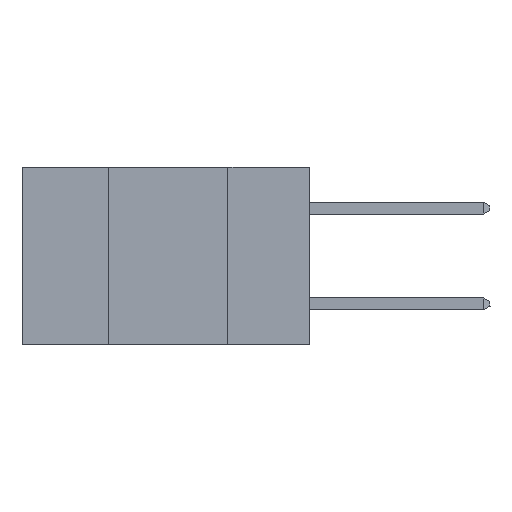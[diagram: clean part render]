
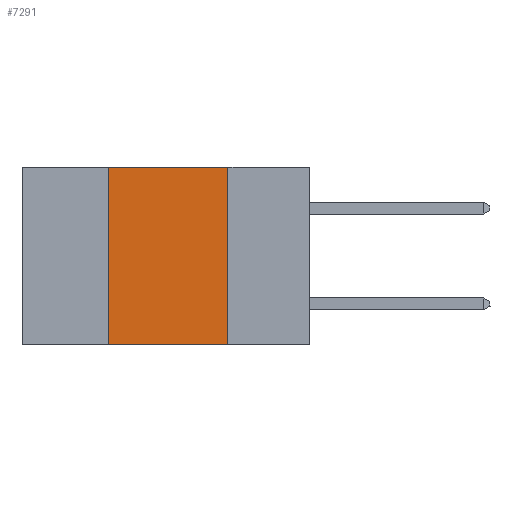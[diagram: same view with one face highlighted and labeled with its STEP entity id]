
A CAD part, left-side view. The second image highlights one B-rep face of the part: STEP entity #7291.
In plain terms, the highlighted planar face has unit normal (-1, 0, 0).
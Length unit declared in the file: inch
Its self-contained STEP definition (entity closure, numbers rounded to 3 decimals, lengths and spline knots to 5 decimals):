
#72 = AXIS2_PLACEMENT_3D ( 'NONE', #28577, #18499, #19022 ) ;
#2441 = VERTEX_POINT ( 'NONE', #14152 ) ;
#2989 = ORIENTED_EDGE ( 'NONE', *, *, #26535, .T. ) ;
#5085 = LINE ( 'NONE', #9541, #8541 ) ;
#5310 = DIRECTION ( 'NONE',  ( 0., -1., 0. ) ) ;
#5740 = VERTEX_POINT ( 'NONE', #23382 ) ;
#6994 = EDGE_CURVE ( 'NONE', #11502, #2441, #5085, .T. ) ;
#7291 = ADVANCED_FACE ( 'NONE', ( #26957 ), #26006, .F. ) ;
#7890 = LINE ( 'NONE', #20004, #15996 ) ;
#7970 = VECTOR ( 'NONE', #14049, 39.37008 ) ;
#8541 = VECTOR ( 'NONE', #21970, 39.37008 ) ;
#9541 = CARTESIAN_POINT ( 'NONE',  ( 0., 0.17, 0. ) ) ;
#9590 = VECTOR ( 'NONE', #28060, 39.37008 ) ;
#10100 = CARTESIAN_POINT ( 'NONE',  ( 0., 0.42, 0. ) ) ;
#11502 = VERTEX_POINT ( 'NONE', #21908 ) ;
#11761 = ORIENTED_EDGE ( 'NONE', *, *, #6994, .F. ) ;
#12871 = EDGE_LOOP ( 'NONE', ( #11761, #29913, #15161, #2989 ) ) ;
#13013 = LINE ( 'NONE', #10100, #9590 ) ;
#14049 = DIRECTION ( 'NONE',  ( 0., -1., 0. ) ) ;
#14152 = CARTESIAN_POINT ( 'NONE',  ( 0., 0.17, -0.37 ) ) ;
#15161 = ORIENTED_EDGE ( 'NONE', *, *, #21247, .F. ) ;
#15996 = VECTOR ( 'NONE', #5310, 39.37008 ) ;
#16060 = EDGE_CURVE ( 'NONE', #5740, #11502, #7890, .T. ) ;
#17569 = VERTEX_POINT ( 'NONE', #21531 ) ;
#18499 = DIRECTION ( 'NONE',  ( 1., 0., 0. ) ) ;
#19022 = DIRECTION ( 'NONE',  ( 0., 0., -1. ) ) ;
#20004 = CARTESIAN_POINT ( 'NONE',  ( 0., 0.6, 0. ) ) ;
#21247 = EDGE_CURVE ( 'NONE', #17569, #5740, #13013, .T. ) ;
#21531 = CARTESIAN_POINT ( 'NONE',  ( 0., 0.42, -0.37 ) ) ;
#21908 = CARTESIAN_POINT ( 'NONE',  ( 0., 0.17, 0. ) ) ;
#21970 = DIRECTION ( 'NONE',  ( 0., 0., -1. ) ) ;
#23382 = CARTESIAN_POINT ( 'NONE',  ( 0., 0.42, 0. ) ) ;
#26006 = PLANE ( 'NONE',  #72 ) ;
#26535 = EDGE_CURVE ( 'NONE', #17569, #2441, #28730, .T. ) ;
#26578 = CARTESIAN_POINT ( 'NONE',  ( 0., 0.6, -0.37 ) ) ;
#26957 = FACE_OUTER_BOUND ( 'NONE', #12871, .T. ) ;
#28060 = DIRECTION ( 'NONE',  ( 0., 0., 1. ) ) ;
#28577 = CARTESIAN_POINT ( 'NONE',  ( 0., 0.6, 0. ) ) ;
#28730 = LINE ( 'NONE', #26578, #7970 ) ;
#29913 = ORIENTED_EDGE ( 'NONE', *, *, #16060, .F. ) ;
